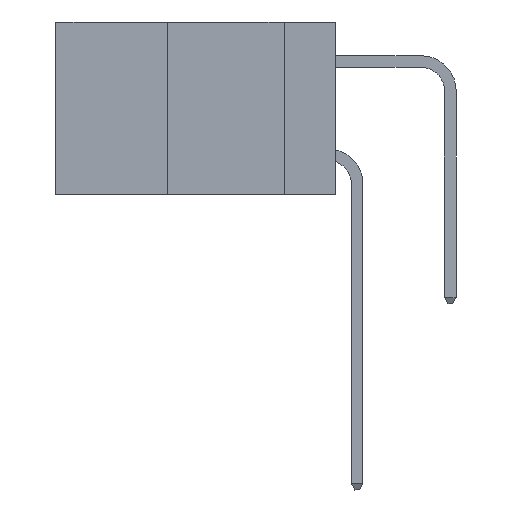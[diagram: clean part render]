
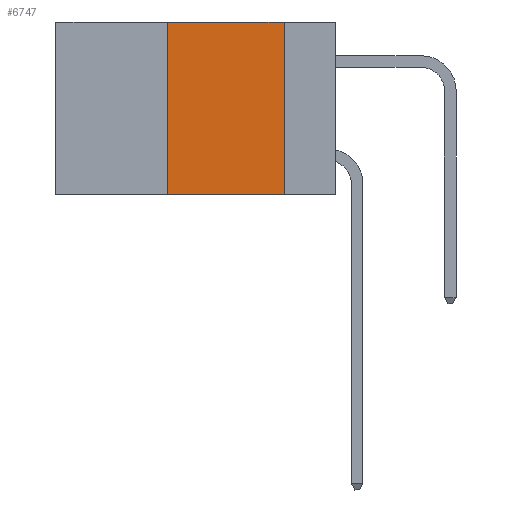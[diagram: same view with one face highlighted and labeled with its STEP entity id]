
A CAD part, left-side view. The second image highlights one B-rep face of the part: STEP entity #6747.
In plain terms, the highlighted planar face has unit normal (-1, 0, 0).
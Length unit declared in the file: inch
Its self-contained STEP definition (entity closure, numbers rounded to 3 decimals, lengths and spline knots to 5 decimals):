
#363 = CARTESIAN_POINT ( 'NONE',  ( 0., 0.6, 0. ) ) ;
#1079 = VERTEX_POINT ( 'NONE', #2408 ) ;
#1191 = CARTESIAN_POINT ( 'NONE',  ( 0., 0.11, 0. ) ) ;
#1790 = VERTEX_POINT ( 'NONE', #15555 ) ;
#1821 = CARTESIAN_POINT ( 'NONE',  ( 0., 0.6, 0. ) ) ;
#2387 = LINE ( 'NONE', #363, #18530 ) ;
#2408 = CARTESIAN_POINT ( 'NONE',  ( 0., 0.11, -0.37 ) ) ;
#2641 = VERTEX_POINT ( 'NONE', #12756 ) ;
#3422 = LINE ( 'NONE', #5569, #7132 ) ;
#3683 = EDGE_CURVE ( 'NONE', #1790, #12695, #2387, .T. ) ;
#4286 = FACE_OUTER_BOUND ( 'NONE', #10641, .T. ) ;
#5138 = DIRECTION ( 'NONE',  ( 1., 0., 0. ) ) ;
#5474 = ORIENTED_EDGE ( 'NONE', *, *, #3683, .F. ) ;
#5569 = CARTESIAN_POINT ( 'NONE',  ( 0., 0.6, -0.37 ) ) ;
#5804 = EDGE_CURVE ( 'NONE', #12695, #1079, #5838, .T. ) ;
#5838 = LINE ( 'NONE', #1191, #13122 ) ;
#6747 = ADVANCED_FACE ( 'NONE', ( #4286 ), #14432, .F. ) ;
#7132 = VECTOR ( 'NONE', #8196, 39.37008 ) ;
#7688 = ORIENTED_EDGE ( 'NONE', *, *, #13715, .T. ) ;
#8196 = DIRECTION ( 'NONE',  ( 0., -1., 0. ) ) ;
#8632 = CARTESIAN_POINT ( 'NONE',  ( 0., 0.11, 0. ) ) ;
#9030 = CARTESIAN_POINT ( 'NONE',  ( 0., 0.36, 0. ) ) ;
#9075 = LINE ( 'NONE', #9030, #13725 ) ;
#10093 = AXIS2_PLACEMENT_3D ( 'NONE', #1821, #5138, #15992 ) ;
#10641 = EDGE_LOOP ( 'NONE', ( #15922, #5474, #15242, #7688 ) ) ;
#10663 = EDGE_CURVE ( 'NONE', #2641, #1790, #9075, .T. ) ;
#12695 = VERTEX_POINT ( 'NONE', #8632 ) ;
#12756 = CARTESIAN_POINT ( 'NONE',  ( 0., 0.36, -0.37 ) ) ;
#13122 = VECTOR ( 'NONE', #16987, 39.37008 ) ;
#13715 = EDGE_CURVE ( 'NONE', #2641, #1079, #3422, .T. ) ;
#13725 = VECTOR ( 'NONE', #19900, 39.37008 ) ;
#14432 = PLANE ( 'NONE',  #10093 ) ;
#15242 = ORIENTED_EDGE ( 'NONE', *, *, #10663, .F. ) ;
#15555 = CARTESIAN_POINT ( 'NONE',  ( 0., 0.36, 0. ) ) ;
#15922 = ORIENTED_EDGE ( 'NONE', *, *, #5804, .F. ) ;
#15992 = DIRECTION ( 'NONE',  ( 0., 0., -1. ) ) ;
#16987 = DIRECTION ( 'NONE',  ( 0., 0., -1. ) ) ;
#18530 = VECTOR ( 'NONE', #20040, 39.37008 ) ;
#19900 = DIRECTION ( 'NONE',  ( 0., 0., 1. ) ) ;
#20040 = DIRECTION ( 'NONE',  ( 0., -1., 0. ) ) ;
